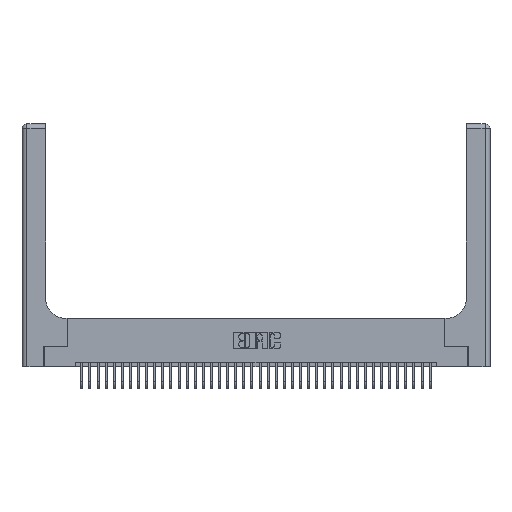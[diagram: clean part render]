
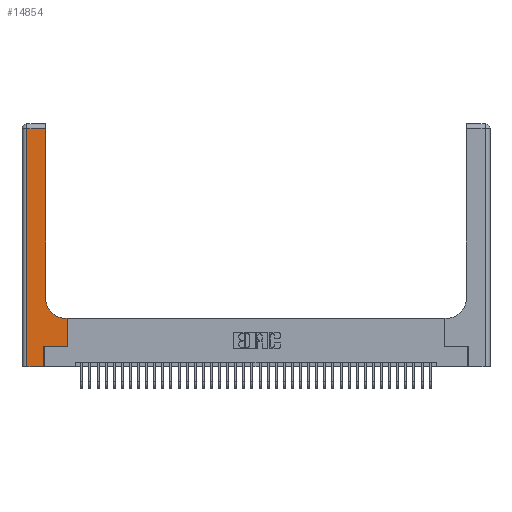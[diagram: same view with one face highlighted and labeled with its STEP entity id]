
A CAD part, top view. The second image highlights one B-rep face of the part: STEP entity #14854.
In plain terms, the highlighted planar face has unit normal (0, 0, 1).
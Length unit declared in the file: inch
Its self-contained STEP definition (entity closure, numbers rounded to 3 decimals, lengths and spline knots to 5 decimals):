
#284 = EDGE_CURVE ( 'NONE', #15810, #29607, #28605, .T. ) ;
#1143 = CARTESIAN_POINT ( 'NONE',  ( 0.5585, 0.6, 0.37 ) ) ;
#1468 = FACE_OUTER_BOUND ( 'NONE', #18056, .T. ) ;
#2355 = AXIS2_PLACEMENT_3D ( 'NONE', #12247, #30022, #12367 ) ;
#3024 = DIRECTION ( 'NONE',  ( 1., 0., 0. ) ) ;
#3805 = EDGE_CURVE ( 'NONE', #35961, #32260, #20993, .T. ) ;
#4542 = EDGE_CURVE ( 'NONE', #32260, #8628, #5282, .T. ) ;
#5007 = DIRECTION ( 'NONE',  ( 0., 1., 0. ) ) ;
#5282 = LINE ( 'NONE', #23779, #35676 ) ;
#5736 = CARTESIAN_POINT ( 'NONE',  ( 0.5415, 0.6, 0.37 ) ) ;
#6257 = VECTOR ( 'NONE', #3024, 39.37008 ) ;
#6650 = VECTOR ( 'NONE', #33185, 39.37008 ) ;
#8234 = VECTOR ( 'NONE', #30081, 39.37008 ) ;
#8479 = EDGE_CURVE ( 'NONE', #12502, #13420, #26540, .T. ) ;
#8628 = VERTEX_POINT ( 'NONE', #26495 ) ;
#9269 = ORIENTED_EDGE ( 'NONE', *, *, #28465, .T. ) ;
#9392 = PLANE ( 'NONE',  #2355 ) ;
#9524 = EDGE_CURVE ( 'NONE', #13420, #15810, #13059, .T. ) ;
#11369 = CARTESIAN_POINT ( 'NONE',  ( 0.269, 0., 0.37 ) ) ;
#11605 = LINE ( 'NONE', #29921, #25429 ) ;
#12134 = DIRECTION ( 'NONE',  ( 0., 1., 0. ) ) ;
#12247 = CARTESIAN_POINT ( 'NONE',  ( 0., 3., 0.37 ) ) ;
#12367 = DIRECTION ( 'NONE',  ( -1., 0., 0. ) ) ;
#12502 = VERTEX_POINT ( 'NONE', #19451 ) ;
#12609 = CARTESIAN_POINT ( 'NONE',  ( 0.269, 0.25, 0.37 ) ) ;
#13059 = LINE ( 'NONE', #37830, #20902 ) ;
#13420 = VERTEX_POINT ( 'NONE', #1143 ) ;
#13644 = CARTESIAN_POINT ( 'NONE',  ( 0.5415, 0.85, 0.37 ) ) ;
#14575 = EDGE_CURVE ( 'NONE', #8628, #12502, #19428, .T. ) ;
#14778 = ORIENTED_EDGE ( 'NONE', *, *, #3805, .T. ) ;
#14808 = ORIENTED_EDGE ( 'NONE', *, *, #4542, .T. ) ;
#14854 = ADVANCED_FACE ( 'NONE', ( #1468 ), #9392, .F. ) ;
#15810 = VERTEX_POINT ( 'NONE', #5736 ) ;
#16594 = DIRECTION ( 'NONE',  ( 1., 0., 0. ) ) ;
#17622 = ORIENTED_EDGE ( 'NONE', *, *, #14575, .T. ) ;
#17903 = LINE ( 'NONE', #35969, #8234 ) ;
#18056 = EDGE_LOOP ( 'NONE', ( #31971, #9269, #18478, #14778, #14808, #17622, #33636, #32176, #23310 ) ) ;
#18478 = ORIENTED_EDGE ( 'NONE', *, *, #22126, .T. ) ;
#18668 = VECTOR ( 'NONE', #5007, 39.37008 ) ;
#19428 = LINE ( 'NONE', #12609, #26374 ) ;
#19451 = CARTESIAN_POINT ( 'NONE',  ( 0.5585, 0.25, 0.37 ) ) ;
#19492 = CARTESIAN_POINT ( 'NONE',  ( 0.2915, 2.94, 0.37 ) ) ;
#20198 = DIRECTION ( 'NONE',  ( -1., 0., 0. ) ) ;
#20902 = VECTOR ( 'NONE', #20198, 39.37008 ) ;
#20993 = LINE ( 'NONE', #35320, #6257 ) ;
#21484 = CARTESIAN_POINT ( 'NONE',  ( 0.06, 0., 0.37 ) ) ;
#22126 = EDGE_CURVE ( 'NONE', #30539, #35961, #17903, .T. ) ;
#22340 = LINE ( 'NONE', #30237, #6650 ) ;
#23310 = ORIENTED_EDGE ( 'NONE', *, *, #284, .T. ) ;
#23779 = CARTESIAN_POINT ( 'NONE',  ( 0.269, 0., 0.37 ) ) ;
#25429 = VECTOR ( 'NONE', #12134, 39.37008 ) ;
#26374 = VECTOR ( 'NONE', #33227, 39.37008 ) ;
#26495 = CARTESIAN_POINT ( 'NONE',  ( 0.269, 0.25, 0.37 ) ) ;
#26540 = LINE ( 'NONE', #37289, #18668 ) ;
#26767 = DIRECTION ( 'NONE',  ( 0., 1., 0. ) ) ;
#28465 = EDGE_CURVE ( 'NONE', #29443, #30539, #22340, .T. ) ;
#28605 = CIRCLE ( 'NONE', #36508, 0.25 ) ;
#29443 = VERTEX_POINT ( 'NONE', #19492 ) ;
#29607 = VERTEX_POINT ( 'NONE', #37903 ) ;
#29921 = CARTESIAN_POINT ( 'NONE',  ( 0.2915, 3., 0.37 ) ) ;
#30007 = CARTESIAN_POINT ( 'NONE',  ( 0.06, 2.94, 0.37 ) ) ;
#30022 = DIRECTION ( 'NONE',  ( 0., 0., -1. ) ) ;
#30081 = DIRECTION ( 'NONE',  ( 0., -1., 0. ) ) ;
#30237 = CARTESIAN_POINT ( 'NONE',  ( 0., 2.94, 0.37 ) ) ;
#30539 = VERTEX_POINT ( 'NONE', #30007 ) ;
#31971 = ORIENTED_EDGE ( 'NONE', *, *, #37200, .T. ) ;
#32176 = ORIENTED_EDGE ( 'NONE', *, *, #9524, .T. ) ;
#32260 = VERTEX_POINT ( 'NONE', #11369 ) ;
#33185 = DIRECTION ( 'NONE',  ( -1., 0., 0. ) ) ;
#33227 = DIRECTION ( 'NONE',  ( 1., 0., 0. ) ) ;
#33636 = ORIENTED_EDGE ( 'NONE', *, *, #8479, .T. ) ;
#34251 = DIRECTION ( 'NONE',  ( 0., 0., -1. ) ) ;
#35320 = CARTESIAN_POINT ( 'NONE',  ( 0., 0., 0.37 ) ) ;
#35676 = VECTOR ( 'NONE', #26767, 39.37008 ) ;
#35961 = VERTEX_POINT ( 'NONE', #21484 ) ;
#35969 = CARTESIAN_POINT ( 'NONE',  ( 0.06, 3., 0.37 ) ) ;
#36508 = AXIS2_PLACEMENT_3D ( 'NONE', #13644, #34251, #16594 ) ;
#37200 = EDGE_CURVE ( 'NONE', #29607, #29443, #11605, .T. ) ;
#37289 = CARTESIAN_POINT ( 'NONE',  ( 0.5585, 0.25, 0.37 ) ) ;
#37830 = CARTESIAN_POINT ( 'NONE',  ( 0.2915, 0.6, 0.37 ) ) ;
#37903 = CARTESIAN_POINT ( 'NONE',  ( 0.2915, 0.85, 0.37 ) ) ;
